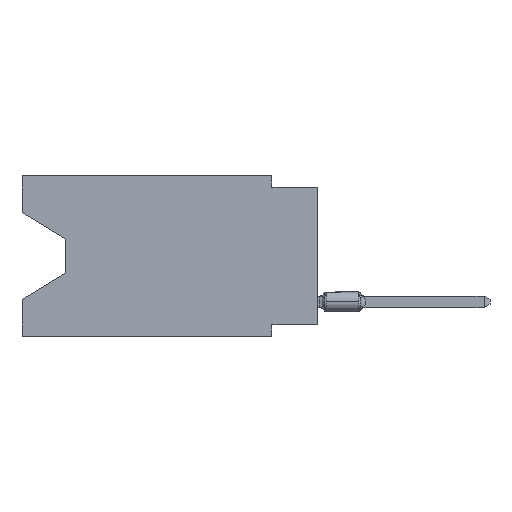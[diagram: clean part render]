
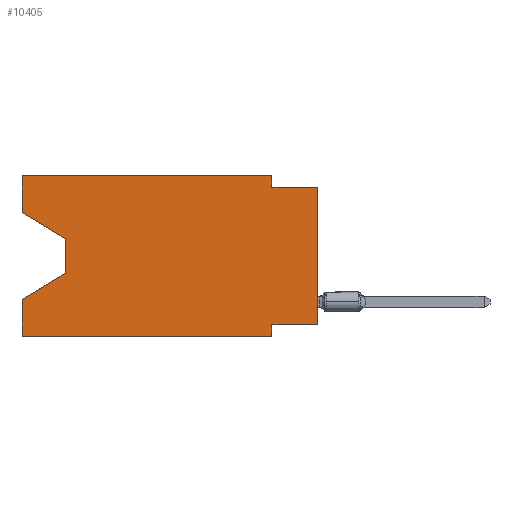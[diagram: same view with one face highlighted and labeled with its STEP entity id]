
A CAD part, left-side view. The second image highlights one B-rep face of the part: STEP entity #10405.
In plain terms, the highlighted planar face has unit normal (-1, 0, 0).
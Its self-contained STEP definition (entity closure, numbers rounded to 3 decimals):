
#224 = EDGE_CURVE ( 'NONE', #2174, #6009, #8525, .T. ) ;
#848 = DIRECTION ( 'NONE',  ( 0., -1., 0. ) ) ;
#1128 = VECTOR ( 'NONE', #3548, 1000. ) ;
#1562 = VERTEX_POINT ( 'NONE', #2739 ) ;
#2174 = VERTEX_POINT ( 'NONE', #3153 ) ;
#2284 = EDGE_CURVE ( 'NONE', #12242, #2401, #17169, .T. ) ;
#2331 = LINE ( 'NONE', #17452, #4719 ) ;
#2373 = EDGE_CURVE ( 'NONE', #6009, #18659, #5826, .T. ) ;
#2401 = VERTEX_POINT ( 'NONE', #19446 ) ;
#2467 = DIRECTION ( 'NONE',  ( 0., 0., -1. ) ) ;
#2739 = CARTESIAN_POINT ( 'NONE',  ( 0., 2.54, -8.89 ) ) ;
#2751 = DIRECTION ( 'NONE',  ( 0., 0., 1. ) ) ;
#2776 = DIRECTION ( 'NONE',  ( 1., 0., 0. ) ) ;
#2787 = CARTESIAN_POINT ( 'NONE',  ( 0., 2.54, -0.635 ) ) ;
#3153 = CARTESIAN_POINT ( 'NONE',  ( 0., 16.383, 0. ) ) ;
#3219 = EDGE_CURVE ( 'NONE', #6165, #1562, #17684, .T. ) ;
#3414 = VECTOR ( 'NONE', #13314, 1000. ) ;
#3548 = DIRECTION ( 'NONE',  ( 0., -0.855, -0.519 ) ) ;
#3731 = CARTESIAN_POINT ( 'NONE',  ( 0., 16.383, -2.038 ) ) ;
#3745 = DIRECTION ( 'NONE',  ( 0., 0.855, -0.519 ) ) ;
#3877 = ORIENTED_EDGE ( 'NONE', *, *, #12240, .T. ) ;
#3936 = LINE ( 'NONE', #8238, #6253 ) ;
#4110 = LINE ( 'NONE', #10214, #12931 ) ;
#4119 = VECTOR ( 'NONE', #13706, 1000. ) ;
#4564 = PLANE ( 'NONE',  #18325 ) ;
#4719 = VECTOR ( 'NONE', #848, 1000. ) ;
#5068 = CARTESIAN_POINT ( 'NONE',  ( 0., 0., -0.635 ) ) ;
#5141 = LINE ( 'NONE', #6827, #8433 ) ;
#5203 = EDGE_CURVE ( 'NONE', #12242, #2174, #4110, .T. ) ;
#5628 = VERTEX_POINT ( 'NONE', #5068 ) ;
#5725 = CARTESIAN_POINT ( 'NONE',  ( 0., 2.54, 0. ) ) ;
#5756 = DIRECTION ( 'NONE',  ( 0., 0., 1. ) ) ;
#5826 = LINE ( 'NONE', #5725, #11309 ) ;
#5857 = FACE_OUTER_BOUND ( 'NONE', #15194, .T. ) ;
#5969 = EDGE_CURVE ( 'NONE', #6746, #11384, #5141, .T. ) ;
#6009 = VERTEX_POINT ( 'NONE', #11123 ) ;
#6165 = VERTEX_POINT ( 'NONE', #11607 ) ;
#6253 = VECTOR ( 'NONE', #11229, 1000. ) ;
#6746 = VERTEX_POINT ( 'NONE', #13749 ) ;
#6827 = CARTESIAN_POINT ( 'NONE',  ( 0., 13.97, -5.385 ) ) ;
#6982 = EDGE_CURVE ( 'NONE', #9529, #5628, #10558, .T. ) ;
#7213 = EDGE_CURVE ( 'NONE', #9529, #6165, #3936, .T. ) ;
#7261 = CARTESIAN_POINT ( 'NONE',  ( 0., 0., 0. ) ) ;
#7266 = CARTESIAN_POINT ( 'NONE',  ( 0., 16.383, -8.89 ) ) ;
#7304 = ORIENTED_EDGE ( 'NONE', *, *, #2373, .F. ) ;
#7535 = VECTOR ( 'NONE', #2467, 1000. ) ;
#7906 = CARTESIAN_POINT ( 'NONE',  ( 0., 16.383, -6.852 ) ) ;
#8238 = CARTESIAN_POINT ( 'NONE',  ( 0., 0., -8.255 ) ) ;
#8433 = VECTOR ( 'NONE', #3745, 1000. ) ;
#8525 = LINE ( 'NONE', #19146, #8660 ) ;
#8660 = VECTOR ( 'NONE', #11221, 1000. ) ;
#8731 = CARTESIAN_POINT ( 'NONE',  ( 0., 0., -8.255 ) ) ;
#8858 = DIRECTION ( 'NONE',  ( 0., 0., -1. ) ) ;
#9435 = ORIENTED_EDGE ( 'NONE', *, *, #224, .F. ) ;
#9529 = VERTEX_POINT ( 'NONE', #8731 ) ;
#9740 = CARTESIAN_POINT ( 'NONE',  ( 0., 16.383, -2.038 ) ) ;
#10214 = CARTESIAN_POINT ( 'NONE',  ( 0., 16.383, 0. ) ) ;
#10385 = VECTOR ( 'NONE', #5756, 1000. ) ;
#10405 = ADVANCED_FACE ( 'NONE', ( #5857 ), #4564, .F. ) ;
#10558 = LINE ( 'NONE', #7261, #10385 ) ;
#10641 = CARTESIAN_POINT ( 'NONE',  ( 0., 16.383, 0. ) ) ;
#10788 = EDGE_CURVE ( 'NONE', #11549, #11384, #19458, .T. ) ;
#10895 = EDGE_CURVE ( 'NONE', #18659, #5628, #11915, .T. ) ;
#10960 = ORIENTED_EDGE ( 'NONE', *, *, #10788, .F. ) ;
#11076 = ORIENTED_EDGE ( 'NONE', *, *, #3219, .F. ) ;
#11123 = CARTESIAN_POINT ( 'NONE',  ( 0., 2.54, 0. ) ) ;
#11221 = DIRECTION ( 'NONE',  ( 0., -1., 0. ) ) ;
#11229 = DIRECTION ( 'NONE',  ( 0., 1., 0. ) ) ;
#11309 = VECTOR ( 'NONE', #13195, 1000. ) ;
#11384 = VERTEX_POINT ( 'NONE', #7906 ) ;
#11549 = VERTEX_POINT ( 'NONE', #7266 ) ;
#11607 = CARTESIAN_POINT ( 'NONE',  ( 0., 2.54, -8.255 ) ) ;
#11915 = LINE ( 'NONE', #19260, #3414 ) ;
#11992 = ORIENTED_EDGE ( 'NONE', *, *, #7213, .F. ) ;
#12019 = LINE ( 'NONE', #13507, #4119 ) ;
#12136 = CARTESIAN_POINT ( 'NONE',  ( 0., 16.383, 0. ) ) ;
#12240 = EDGE_CURVE ( 'NONE', #11549, #1562, #2331, .T. ) ;
#12242 = VERTEX_POINT ( 'NONE', #3731 ) ;
#12470 = ORIENTED_EDGE ( 'NONE', *, *, #16166, .T. ) ;
#12931 = VECTOR ( 'NONE', #19427, 1000. ) ;
#13195 = DIRECTION ( 'NONE',  ( 0., 0., -1. ) ) ;
#13314 = DIRECTION ( 'NONE',  ( 0., -1., 0. ) ) ;
#13424 = CARTESIAN_POINT ( 'NONE',  ( 0., 2.54, -8.89 ) ) ;
#13507 = CARTESIAN_POINT ( 'NONE',  ( 0., 13.97, -3.505 ) ) ;
#13539 = ORIENTED_EDGE ( 'NONE', *, *, #6982, .T. ) ;
#13706 = DIRECTION ( 'NONE',  ( 0., 0., -1. ) ) ;
#13749 = CARTESIAN_POINT ( 'NONE',  ( 0., 13.97, -5.385 ) ) ;
#14856 = VECTOR ( 'NONE', #2751, 1000. ) ;
#15194 = EDGE_LOOP ( 'NONE', ( #17190, #12470, #18538, #10960, #3877, #11076, #11992, #13539, #19403, #7304, #9435, #17899 ) ) ;
#16166 = EDGE_CURVE ( 'NONE', #2401, #6746, #12019, .T. ) ;
#17169 = LINE ( 'NONE', #9740, #1128 ) ;
#17190 = ORIENTED_EDGE ( 'NONE', *, *, #2284, .T. ) ;
#17452 = CARTESIAN_POINT ( 'NONE',  ( 0., 16.383, -8.89 ) ) ;
#17684 = LINE ( 'NONE', #13424, #7535 ) ;
#17899 = ORIENTED_EDGE ( 'NONE', *, *, #5203, .F. ) ;
#18325 = AXIS2_PLACEMENT_3D ( 'NONE', #12136, #2776, #8858 ) ;
#18538 = ORIENTED_EDGE ( 'NONE', *, *, #5969, .T. ) ;
#18659 = VERTEX_POINT ( 'NONE', #2787 ) ;
#19146 = CARTESIAN_POINT ( 'NONE',  ( 0., 16.383, 0. ) ) ;
#19260 = CARTESIAN_POINT ( 'NONE',  ( 0., 0., -0.635 ) ) ;
#19403 = ORIENTED_EDGE ( 'NONE', *, *, #10895, .F. ) ;
#19427 = DIRECTION ( 'NONE',  ( 0., 0., 1. ) ) ;
#19446 = CARTESIAN_POINT ( 'NONE',  ( 0., 13.97, -3.505 ) ) ;
#19458 = LINE ( 'NONE', #10641, #14856 ) ;
